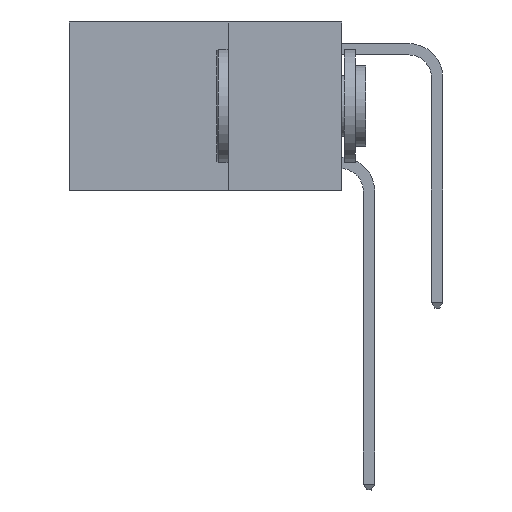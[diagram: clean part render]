
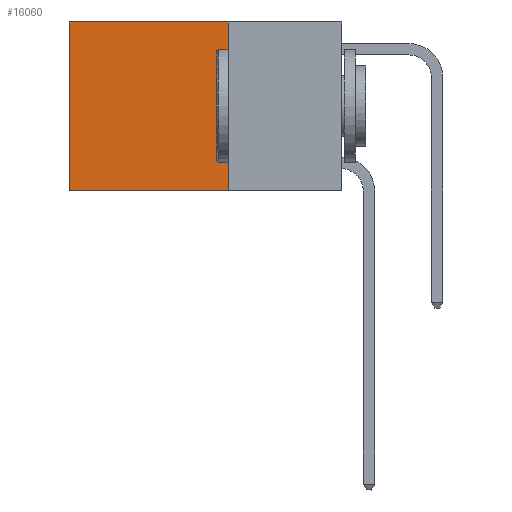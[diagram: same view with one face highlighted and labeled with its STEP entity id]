
A CAD part, left-side view. The second image highlights one B-rep face of the part: STEP entity #16060.
In plain terms, the highlighted planar face has unit normal (-1, 0, 0).
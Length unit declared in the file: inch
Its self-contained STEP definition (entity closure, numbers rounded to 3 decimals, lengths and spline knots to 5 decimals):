
#139 = EDGE_CURVE ( 'NONE', #15376, #21239, #653, .T. ) ;
#193 = DIRECTION ( 'NONE',  ( 0., 1., 0. ) ) ;
#260 = VECTOR ( 'NONE', #17459, 39.37008 ) ;
#653 = LINE ( 'NONE', #8617, #21710 ) ;
#1758 = LINE ( 'NONE', #18843, #12631 ) ;
#2024 = VECTOR ( 'NONE', #7729, 39.37008 ) ;
#3181 = CARTESIAN_POINT ( 'NONE',  ( 0.2625, 0.6, 0. ) ) ;
#4437 = EDGE_LOOP ( 'NONE', ( #17394, #6530, #24990, #10580 ) ) ;
#5181 = PLANE ( 'NONE',  #23493 ) ;
#6530 = ORIENTED_EDGE ( 'NONE', *, *, #15163, .F. ) ;
#7729 = DIRECTION ( 'NONE',  ( 0., 0., -1. ) ) ;
#8617 = CARTESIAN_POINT ( 'NONE',  ( 0.2625, 0.25, 0. ) ) ;
#8622 = DIRECTION ( 'NONE',  ( 0., 1., 0. ) ) ;
#9241 = CARTESIAN_POINT ( 'NONE',  ( 0.2625, 0.25, 0. ) ) ;
#9297 = DIRECTION ( 'NONE',  ( 0., 0., -1. ) ) ;
#9863 = CARTESIAN_POINT ( 'NONE',  ( 0.2625, 0.25, -0.37 ) ) ;
#10580 = ORIENTED_EDGE ( 'NONE', *, *, #139, .T. ) ;
#11873 = CARTESIAN_POINT ( 'NONE',  ( 0.2625, 0.25, 0. ) ) ;
#12631 = VECTOR ( 'NONE', #8622, 39.37008 ) ;
#12659 = CARTESIAN_POINT ( 'NONE',  ( 0.2625, 0.6, -0.37 ) ) ;
#13489 = EDGE_CURVE ( 'NONE', #21239, #25428, #20678, .T. ) ;
#15163 = EDGE_CURVE ( 'NONE', #23865, #25428, #1758, .T. ) ;
#15376 = VERTEX_POINT ( 'NONE', #9241 ) ;
#16060 = ADVANCED_FACE ( 'NONE', ( #18486 ), #5181, .F. ) ;
#17394 = ORIENTED_EDGE ( 'NONE', *, *, #13489, .T. ) ;
#17459 = DIRECTION ( 'NONE',  ( 0., 0., -1. ) ) ;
#17707 = CARTESIAN_POINT ( 'NONE',  ( 0.2625, 0.6, 0. ) ) ;
#18486 = FACE_OUTER_BOUND ( 'NONE', #4437, .T. ) ;
#18843 = CARTESIAN_POINT ( 'NONE',  ( 0.2625, 0.25, -0.37 ) ) ;
#19514 = CARTESIAN_POINT ( 'NONE',  ( 0.2625, 0.25, 0. ) ) ;
#20678 = LINE ( 'NONE', #3181, #260 ) ;
#21239 = VERTEX_POINT ( 'NONE', #17707 ) ;
#21561 = DIRECTION ( 'NONE',  ( 1., 0., 0. ) ) ;
#21710 = VECTOR ( 'NONE', #193, 39.37008 ) ;
#23222 = EDGE_CURVE ( 'NONE', #15376, #23865, #23690, .T. ) ;
#23493 = AXIS2_PLACEMENT_3D ( 'NONE', #19514, #21561, #9297 ) ;
#23690 = LINE ( 'NONE', #11873, #2024 ) ;
#23865 = VERTEX_POINT ( 'NONE', #9863 ) ;
#24990 = ORIENTED_EDGE ( 'NONE', *, *, #23222, .F. ) ;
#25428 = VERTEX_POINT ( 'NONE', #12659 ) ;
